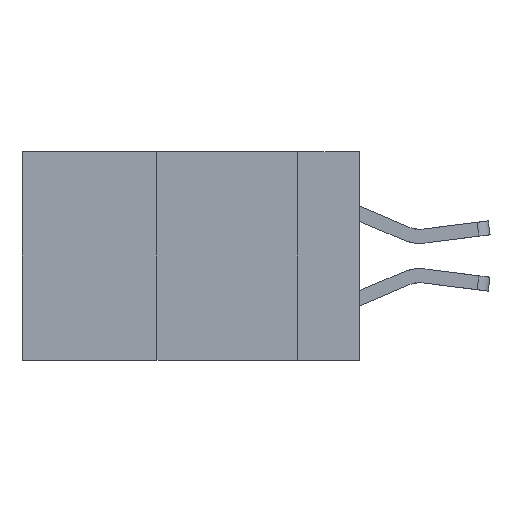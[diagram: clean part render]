
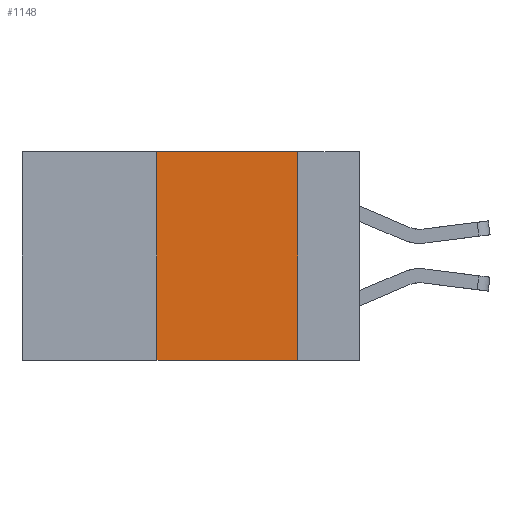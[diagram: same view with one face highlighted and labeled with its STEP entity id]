
A CAD part, left-side view. The second image highlights one B-rep face of the part: STEP entity #1148.
In plain terms, the highlighted planar face has unit normal (-1, 0, 0).
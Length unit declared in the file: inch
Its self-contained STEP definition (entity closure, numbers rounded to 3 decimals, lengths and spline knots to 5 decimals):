
#770 = VERTEX_POINT ( 'NONE', #10586 ) ;
#1148 = ADVANCED_FACE ( 'NONE', ( #10994 ), #3739, .F. ) ;
#1162 = CARTESIAN_POINT ( 'NONE',  ( 0., 0.36, -0.37 ) ) ;
#1405 = VECTOR ( 'NONE', #1688, 39.37008 ) ;
#1627 = AXIS2_PLACEMENT_3D ( 'NONE', #12613, #11175, #7611 ) ;
#1688 = DIRECTION ( 'NONE',  ( 0., -1., 0. ) ) ;
#3152 = ORIENTED_EDGE ( 'NONE', *, *, #3428, .T. ) ;
#3428 = EDGE_CURVE ( 'NONE', #3857, #770, #8337, .T. ) ;
#3608 = DIRECTION ( 'NONE',  ( 0., 0., -1. ) ) ;
#3739 = PLANE ( 'NONE',  #1627 ) ;
#3857 = VERTEX_POINT ( 'NONE', #1162 ) ;
#5727 = EDGE_CURVE ( 'NONE', #15262, #770, #11036, .T. ) ;
#6420 = VECTOR ( 'NONE', #12514, 39.37008 ) ;
#7611 = DIRECTION ( 'NONE',  ( 0., 0., -1. ) ) ;
#8337 = LINE ( 'NONE', #11718, #1405 ) ;
#8442 = ORIENTED_EDGE ( 'NONE', *, *, #12042, .F. ) ;
#8701 = CARTESIAN_POINT ( 'NONE',  ( 0., 0.11, 0. ) ) ;
#9999 = DIRECTION ( 'NONE',  ( 0., -1., 0. ) ) ;
#10333 = EDGE_CURVE ( 'NONE', #13455, #15262, #14815, .T. ) ;
#10586 = CARTESIAN_POINT ( 'NONE',  ( 0., 0.11, -0.37 ) ) ;
#10623 = EDGE_LOOP ( 'NONE', ( #13513, #13543, #8442, #3152 ) ) ;
#10994 = FACE_OUTER_BOUND ( 'NONE', #10623, .T. ) ;
#11036 = LINE ( 'NONE', #8701, #11241 ) ;
#11175 = DIRECTION ( 'NONE',  ( 1., 0., 0. ) ) ;
#11211 = CARTESIAN_POINT ( 'NONE',  ( 0., 0.6, 0. ) ) ;
#11241 = VECTOR ( 'NONE', #3608, 39.37008 ) ;
#11348 = CARTESIAN_POINT ( 'NONE',  ( 0., 0.36, 0. ) ) ;
#11718 = CARTESIAN_POINT ( 'NONE',  ( 0., 0.6, -0.37 ) ) ;
#12042 = EDGE_CURVE ( 'NONE', #3857, #13455, #15559, .T. ) ;
#12514 = DIRECTION ( 'NONE',  ( 0., 0., 1. ) ) ;
#12613 = CARTESIAN_POINT ( 'NONE',  ( 0., 0.6, 0. ) ) ;
#12640 = VECTOR ( 'NONE', #9999, 39.37008 ) ;
#12641 = CARTESIAN_POINT ( 'NONE',  ( 0., 0.36, 0. ) ) ;
#13455 = VERTEX_POINT ( 'NONE', #12641 ) ;
#13513 = ORIENTED_EDGE ( 'NONE', *, *, #5727, .F. ) ;
#13543 = ORIENTED_EDGE ( 'NONE', *, *, #10333, .F. ) ;
#14454 = CARTESIAN_POINT ( 'NONE',  ( 0., 0.11, 0. ) ) ;
#14815 = LINE ( 'NONE', #11211, #12640 ) ;
#15262 = VERTEX_POINT ( 'NONE', #14454 ) ;
#15559 = LINE ( 'NONE', #11348, #6420 ) ;
